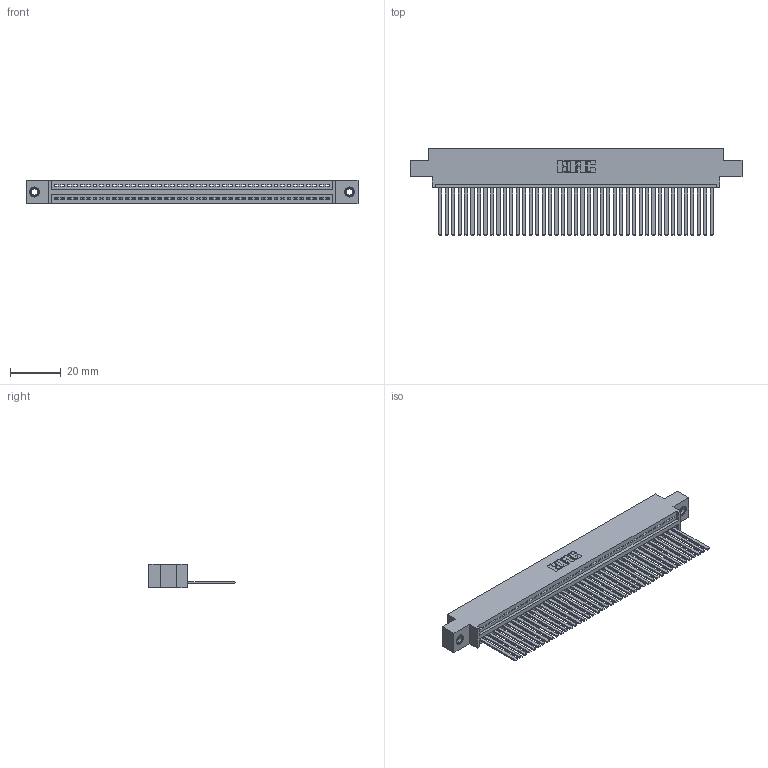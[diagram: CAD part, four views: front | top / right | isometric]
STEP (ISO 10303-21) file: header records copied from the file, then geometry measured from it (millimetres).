
FILE_DESCRIPTION (( 'STEP AP203' ), '1' );
FILE_NAME ('395-043-544-607.STEP', '2018-11-15T16:46:04', ( '' ), ( '' ), 'SwSTEP 2.0', 'SolidWorks 2016', '' );
FILE_SCHEMA (( 'CONFIG_CONTROL_DESIGN' ));
Length unit declared in the file: inch
Products named in the file (4): 345 Part_0.170 Offset - 0.156 Dia-TI; 345-292-001_345-293-144; 395-043-544-607; 345-250-001_345-250-005-103
Assembly tree (46 placements, depth 2):
  395-043-544-607
    345 Part_0.170 Offset - 0.156 Dia-TI
    345-292-001_345-293-144  x43
    345-250-001_345-250-005-103  x2
Bounding box: 130.43 x 33.96 x 9.4 mm (x, y, z)
Volume: 12767.6 mm3; surface area: 18634.7 mm2
Topology: 46 solids, 46 shells, 2426 faces, 7283 edges, 4790 vertices
Faces by surface type: plane 1664, cylinder 746, cone 12, torus 4
Entity records: 33362 total; most frequent: CARTESIAN_POINT 5760, ORIENTED_EDGE 5730, DIRECTION 5053, EDGE_CURVE 2865, VECTOR 2545, LINE 2545, VERTEX_POINT 1904, AXIS2_PLACEMENT_3D 1254
